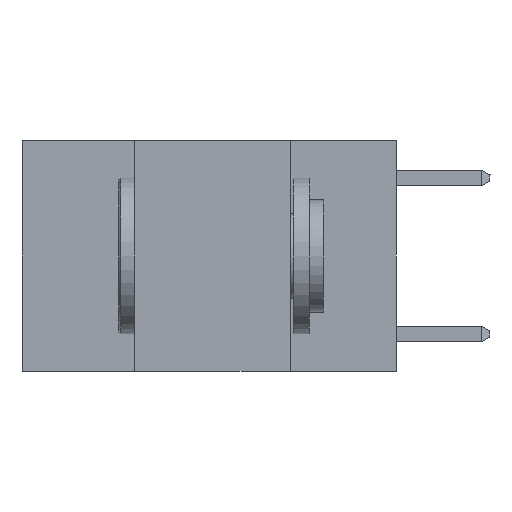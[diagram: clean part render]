
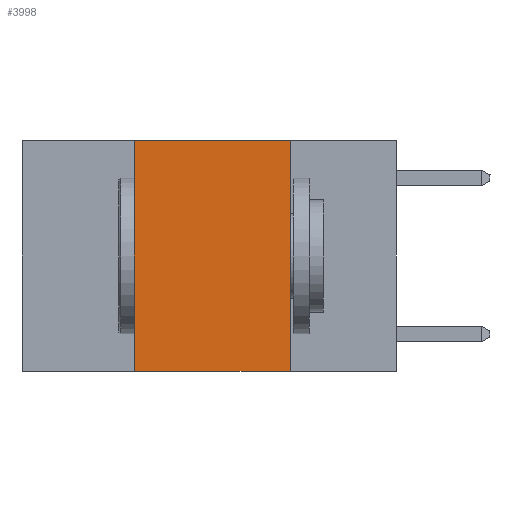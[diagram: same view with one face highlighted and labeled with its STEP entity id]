
A CAD part, left-side view. The second image highlights one B-rep face of the part: STEP entity #3998.
In plain terms, the highlighted planar face has unit normal (-1, 0, 0).
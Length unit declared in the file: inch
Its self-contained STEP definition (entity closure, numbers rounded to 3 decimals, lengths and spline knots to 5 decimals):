
#15 = VERTEX_POINT ( 'NONE', #7943 ) ;
#312 = DIRECTION ( 'NONE',  ( 0., 0., -1. ) ) ;
#988 = EDGE_CURVE ( 'NONE', #9477, #2054, #1328, .T. ) ;
#1279 = CARTESIAN_POINT ( 'NONE',  ( 0., 0.6, 0. ) ) ;
#1328 = LINE ( 'NONE', #8757, #1607 ) ;
#1395 = EDGE_CURVE ( 'NONE', #2054, #7982, #5706, .T. ) ;
#1499 = AXIS2_PLACEMENT_3D ( 'NONE', #1279, #7271, #7319 ) ;
#1549 = ORIENTED_EDGE ( 'NONE', *, *, #2611, .F. ) ;
#1607 = VECTOR ( 'NONE', #5733, 39.37008 ) ;
#1846 = LINE ( 'NONE', #4082, #9162 ) ;
#2025 = CARTESIAN_POINT ( 'NONE',  ( 0., 0.17, 0. ) ) ;
#2030 = DIRECTION ( 'NONE',  ( 0., -1., 0. ) ) ;
#2054 = VERTEX_POINT ( 'NONE', #5204 ) ;
#2611 = EDGE_CURVE ( 'NONE', #7982, #15, #1846, .T. ) ;
#2706 = PLANE ( 'NONE',  #1499 ) ;
#3577 = FACE_OUTER_BOUND ( 'NONE', #5133, .T. ) ;
#3998 = ADVANCED_FACE ( 'NONE', ( #3577 ), #2706, .F. ) ;
#4082 = CARTESIAN_POINT ( 'NONE',  ( 0., 0.17, 0. ) ) ;
#4189 = ORIENTED_EDGE ( 'NONE', *, *, #1395, .F. ) ;
#4203 = ORIENTED_EDGE ( 'NONE', *, *, #988, .F. ) ;
#4511 = CARTESIAN_POINT ( 'NONE',  ( 0., 0.6, -0.37 ) ) ;
#5133 = EDGE_LOOP ( 'NONE', ( #1549, #4189, #4203, #8149 ) ) ;
#5204 = CARTESIAN_POINT ( 'NONE',  ( 0., 0.42, 0. ) ) ;
#5259 = VECTOR ( 'NONE', #5891, 39.37008 ) ;
#5706 = LINE ( 'NONE', #6868, #8518 ) ;
#5733 = DIRECTION ( 'NONE',  ( 0., 0., 1. ) ) ;
#5891 = DIRECTION ( 'NONE',  ( 0., -1., 0. ) ) ;
#6746 = LINE ( 'NONE', #4511, #5259 ) ;
#6868 = CARTESIAN_POINT ( 'NONE',  ( 0., 0.6, 0. ) ) ;
#7271 = DIRECTION ( 'NONE',  ( 1., 0., 0. ) ) ;
#7319 = DIRECTION ( 'NONE',  ( 0., 0., -1. ) ) ;
#7943 = CARTESIAN_POINT ( 'NONE',  ( 0., 0.17, -0.37 ) ) ;
#7982 = VERTEX_POINT ( 'NONE', #2025 ) ;
#8149 = ORIENTED_EDGE ( 'NONE', *, *, #8533, .T. ) ;
#8327 = CARTESIAN_POINT ( 'NONE',  ( 0., 0.42, -0.37 ) ) ;
#8518 = VECTOR ( 'NONE', #2030, 39.37008 ) ;
#8533 = EDGE_CURVE ( 'NONE', #9477, #15, #6746, .T. ) ;
#8757 = CARTESIAN_POINT ( 'NONE',  ( 0., 0.42, 0. ) ) ;
#9162 = VECTOR ( 'NONE', #312, 39.37008 ) ;
#9477 = VERTEX_POINT ( 'NONE', #8327 ) ;
